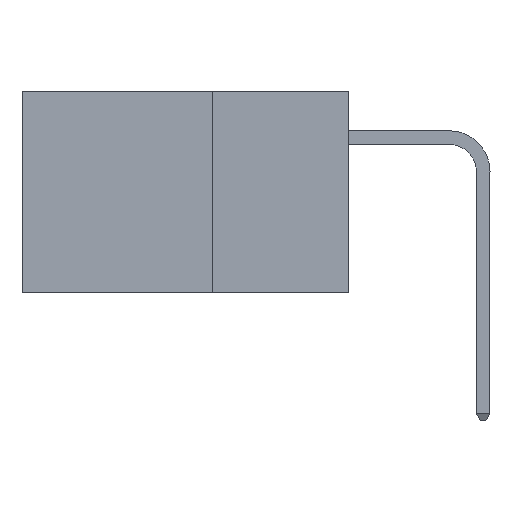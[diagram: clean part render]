
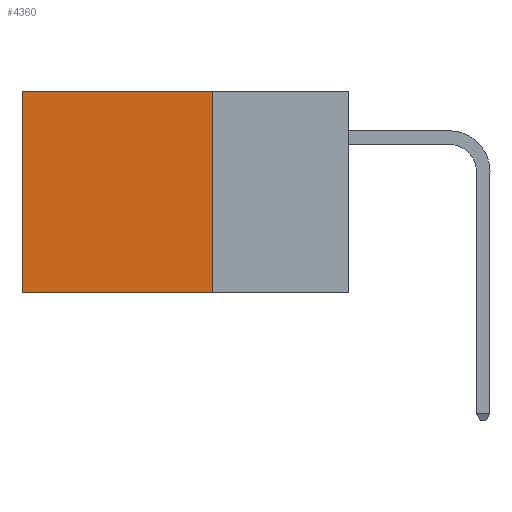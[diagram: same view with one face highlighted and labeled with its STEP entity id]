
A CAD part, left-side view. The second image highlights one B-rep face of the part: STEP entity #4360.
In plain terms, the highlighted planar face has unit normal (-1, 0, 0).
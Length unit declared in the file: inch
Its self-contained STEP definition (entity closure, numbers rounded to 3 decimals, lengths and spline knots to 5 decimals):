
#31 = DIRECTION ( 'NONE',  ( 0., 0., -1. ) ) ;
#836 = EDGE_LOOP ( 'NONE', ( #3168, #6758, #2272, #8000 ) ) ;
#2272 = ORIENTED_EDGE ( 'NONE', *, *, #2923, .F. ) ;
#2277 = DIRECTION ( 'NONE',  ( 0., 1., 0. ) ) ;
#2438 = CARTESIAN_POINT ( 'NONE',  ( 0.2875, 0.25, -0.37 ) ) ;
#2711 = LINE ( 'NONE', #2438, #8067 ) ;
#2787 = VERTEX_POINT ( 'NONE', #7437 ) ;
#2923 = EDGE_CURVE ( 'NONE', #12874, #2787, #7687, .T. ) ;
#3105 = DIRECTION ( 'NONE',  ( 1., 0., 0. ) ) ;
#3168 = ORIENTED_EDGE ( 'NONE', *, *, #8082, .T. ) ;
#4360 = ADVANCED_FACE ( 'NONE', ( #9775 ), #12073, .F. ) ;
#4704 = VECTOR ( 'NONE', #11446, 39.37008 ) ;
#4904 = VECTOR ( 'NONE', #31, 39.37008 ) ;
#5121 = EDGE_CURVE ( 'NONE', #12874, #11940, #5178, .T. ) ;
#5178 = LINE ( 'NONE', #5600, #7637 ) ;
#5600 = CARTESIAN_POINT ( 'NONE',  ( 0.2875, 0.25, 0. ) ) ;
#6273 = CARTESIAN_POINT ( 'NONE',  ( 0.2875, 0.6, -0.37 ) ) ;
#6586 = CARTESIAN_POINT ( 'NONE',  ( 0.2875, 0.25, 0. ) ) ;
#6758 = ORIENTED_EDGE ( 'NONE', *, *, #9741, .F. ) ;
#7437 = CARTESIAN_POINT ( 'NONE',  ( 0.2875, 0.25, -0.37 ) ) ;
#7637 = VECTOR ( 'NONE', #2277, 39.37008 ) ;
#7662 = CARTESIAN_POINT ( 'NONE',  ( 0.2875, 0.6, 0. ) ) ;
#7687 = LINE ( 'NONE', #6586, #4904 ) ;
#8000 = ORIENTED_EDGE ( 'NONE', *, *, #5121, .T. ) ;
#8067 = VECTOR ( 'NONE', #11563, 39.37008 ) ;
#8082 = EDGE_CURVE ( 'NONE', #11940, #9381, #12740, .T. ) ;
#9381 = VERTEX_POINT ( 'NONE', #6273 ) ;
#9383 = CARTESIAN_POINT ( 'NONE',  ( 0.2875, 0.25, 0. ) ) ;
#9741 = EDGE_CURVE ( 'NONE', #2787, #9381, #2711, .T. ) ;
#9775 = FACE_OUTER_BOUND ( 'NONE', #836, .T. ) ;
#9862 = CARTESIAN_POINT ( 'NONE',  ( 0.2875, 0.25, 0. ) ) ;
#10045 = AXIS2_PLACEMENT_3D ( 'NONE', #9383, #3105, #10347 ) ;
#10347 = DIRECTION ( 'NONE',  ( 0., 0., -1. ) ) ;
#11418 = CARTESIAN_POINT ( 'NONE',  ( 0.2875, 0.6, 0. ) ) ;
#11446 = DIRECTION ( 'NONE',  ( 0., 0., -1. ) ) ;
#11563 = DIRECTION ( 'NONE',  ( 0., 1., 0. ) ) ;
#11940 = VERTEX_POINT ( 'NONE', #11418 ) ;
#12073 = PLANE ( 'NONE',  #10045 ) ;
#12740 = LINE ( 'NONE', #7662, #4704 ) ;
#12874 = VERTEX_POINT ( 'NONE', #9862 ) ;
